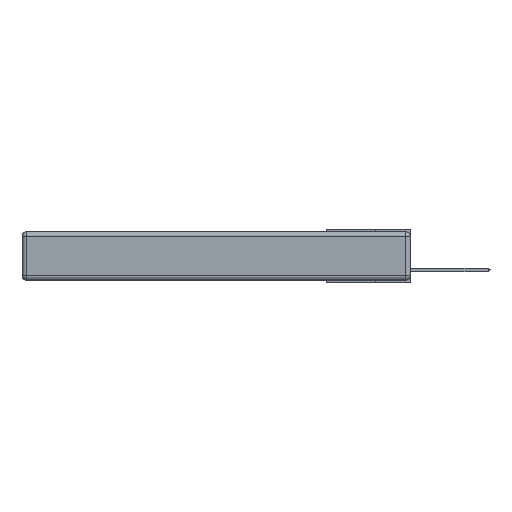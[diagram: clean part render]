
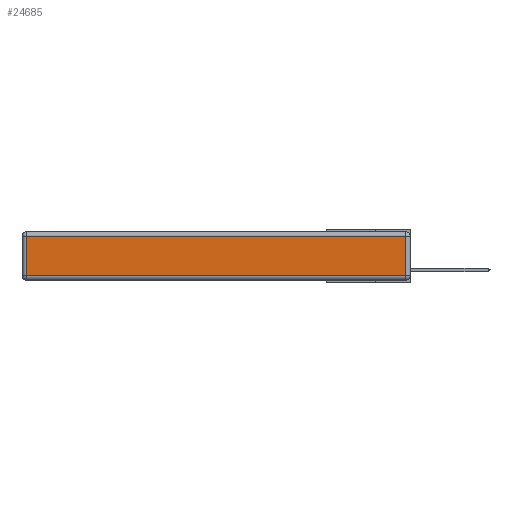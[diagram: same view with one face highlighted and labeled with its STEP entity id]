
A CAD part, left-side view. The second image highlights one B-rep face of the part: STEP entity #24685.
In plain terms, the highlighted planar face has unit normal (-1, 0, 0).
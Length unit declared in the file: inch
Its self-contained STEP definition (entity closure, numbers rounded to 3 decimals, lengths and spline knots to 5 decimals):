
#2468 = CARTESIAN_POINT ( 'NONE',  ( 0., 0.03, -0.03 ) ) ;
#3062 = CARTESIAN_POINT ( 'NONE',  ( 0., 2.75, -0.03 ) ) ;
#4859 = CARTESIAN_POINT ( 'NONE',  ( 0., 2.72, -0.03 ) ) ;
#4946 = FACE_OUTER_BOUND ( 'NONE', #14482, .T. ) ;
#6490 = CARTESIAN_POINT ( 'NONE',  ( 0., 0., -0.343 ) ) ;
#6724 = VERTEX_POINT ( 'NONE', #2468 ) ;
#6903 = LINE ( 'NONE', #26279, #16129 ) ;
#7429 = VERTEX_POINT ( 'NONE', #18163 ) ;
#8188 = ORIENTED_EDGE ( 'NONE', *, *, #28090, .T. ) ;
#8228 = DIRECTION ( 'NONE',  ( 0., 0., -1. ) ) ;
#8383 = DIRECTION ( 'NONE',  ( 0., 0., 1. ) ) ;
#10186 = EDGE_CURVE ( 'NONE', #30212, #7429, #11973, .T. ) ;
#11174 = PLANE ( 'NONE',  #15713 ) ;
#11759 = DIRECTION ( 'NONE',  ( 0., 0., 1. ) ) ;
#11973 = LINE ( 'NONE', #13512, #31719 ) ;
#12711 = VERTEX_POINT ( 'NONE', #16280 ) ;
#13512 = CARTESIAN_POINT ( 'NONE',  ( 0., 2.72, -0.343 ) ) ;
#14249 = LINE ( 'NONE', #23230, #17475 ) ;
#14482 = EDGE_LOOP ( 'NONE', ( #18575, #23184, #8188, #32353 ) ) ;
#15713 = AXIS2_PLACEMENT_3D ( 'NONE', #6490, #21416, #11759 ) ;
#15732 = DIRECTION ( 'NONE',  ( 0., 1., 0. ) ) ;
#16129 = VECTOR ( 'NONE', #8383, 39.37008 ) ;
#16280 = CARTESIAN_POINT ( 'NONE',  ( 0., 0.03, -0.313 ) ) ;
#17475 = VECTOR ( 'NONE', #31118, 39.37008 ) ;
#18163 = CARTESIAN_POINT ( 'NONE',  ( 0., 2.72, -0.313 ) ) ;
#18575 = ORIENTED_EDGE ( 'NONE', *, *, #24345, .T. ) ;
#21416 = DIRECTION ( 'NONE',  ( -1., 0., 0. ) ) ;
#22951 = LINE ( 'NONE', #3062, #26564 ) ;
#23184 = ORIENTED_EDGE ( 'NONE', *, *, #25841, .T. ) ;
#23230 = CARTESIAN_POINT ( 'NONE',  ( 0., 0., -0.313 ) ) ;
#24345 = EDGE_CURVE ( 'NONE', #7429, #12711, #14249, .T. ) ;
#24685 = ADVANCED_FACE ( 'NONE', ( #4946 ), #11174, .T. ) ;
#25841 = EDGE_CURVE ( 'NONE', #12711, #6724, #6903, .T. ) ;
#26279 = CARTESIAN_POINT ( 'NONE',  ( 0., 0.03, -0.343 ) ) ;
#26564 = VECTOR ( 'NONE', #15732, 39.37008 ) ;
#28090 = EDGE_CURVE ( 'NONE', #6724, #30212, #22951, .T. ) ;
#30212 = VERTEX_POINT ( 'NONE', #4859 ) ;
#31118 = DIRECTION ( 'NONE',  ( 0., -1., 0. ) ) ;
#31719 = VECTOR ( 'NONE', #8228, 39.37008 ) ;
#32353 = ORIENTED_EDGE ( 'NONE', *, *, #10186, .T. ) ;
